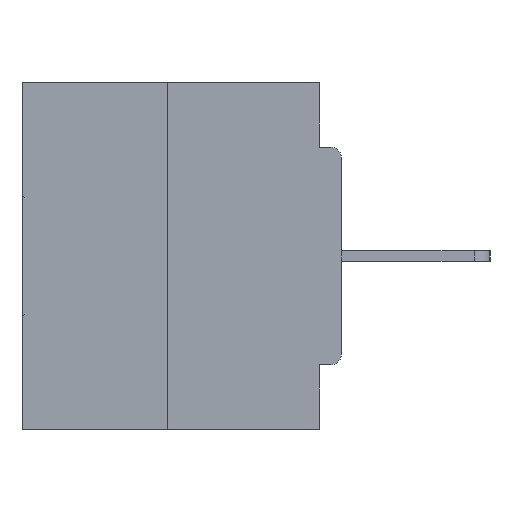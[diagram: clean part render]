
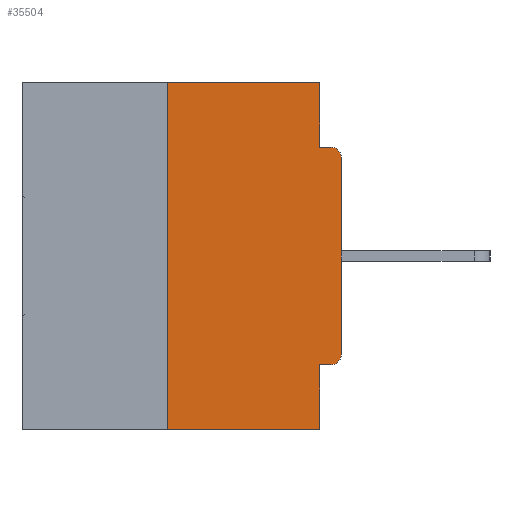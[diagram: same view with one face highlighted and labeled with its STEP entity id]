
A CAD part, left-side view. The second image highlights one B-rep face of the part: STEP entity #35504.
In plain terms, the highlighted planar face has unit normal (-1, 0, 0).
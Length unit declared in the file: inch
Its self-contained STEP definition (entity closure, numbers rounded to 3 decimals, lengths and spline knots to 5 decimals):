
#377 = VECTOR ( 'NONE', #14515, 39.37008 ) ;
#381 = EDGE_CURVE ( 'NONE', #32052, #748, #25562, .T. ) ;
#748 = VERTEX_POINT ( 'NONE', #15202 ) ;
#907 = VERTEX_POINT ( 'NONE', #24732 ) ;
#1870 = ORIENTED_EDGE ( 'NONE', *, *, #14943, .F. ) ;
#2485 = VECTOR ( 'NONE', #12413, 39.37008 ) ;
#2733 = ORIENTED_EDGE ( 'NONE', *, *, #22326, .F. ) ;
#3376 = VECTOR ( 'NONE', #28924, 39.37008 ) ;
#3821 = CARTESIAN_POINT ( 'NONE',  ( 0., 0.015, -0.3915 ) ) ;
#4002 = DIRECTION ( 'NONE',  ( 1., 0., 0. ) ) ;
#4082 = EDGE_CURVE ( 'NONE', #11433, #25136, #16885, .T. ) ;
#5903 = CARTESIAN_POINT ( 'NONE',  ( 0., 0.031, -0.0935 ) ) ;
#6406 = VERTEX_POINT ( 'NONE', #17067 ) ;
#6775 = DIRECTION ( 'NONE',  ( 0., 0., -1. ) ) ;
#7288 = EDGE_CURVE ( 'NONE', #907, #22266, #7903, .T. ) ;
#7825 = ORIENTED_EDGE ( 'NONE', *, *, #21846, .F. ) ;
#7903 = CIRCLE ( 'NONE', #11934, 0.015 ) ;
#8400 = DIRECTION ( 'NONE',  ( 0., -1., 0. ) ) ;
#8404 = ORIENTED_EDGE ( 'NONE', *, *, #32680, .T. ) ;
#8707 = LINE ( 'NONE', #10869, #33222 ) ;
#8786 = CIRCLE ( 'NONE', #23450, 0.015 ) ;
#9446 = EDGE_LOOP ( 'NONE', ( #37067, #15002, #9906, #2733, #30950, #36759, #8404, #12024, #1870, #7825 ) ) ;
#9605 = LINE ( 'NONE', #28944, #32322 ) ;
#9755 = EDGE_CURVE ( 'NONE', #11433, #32052, #9605, .T. ) ;
#9899 = CARTESIAN_POINT ( 'NONE',  ( 0., 0.46, 0. ) ) ;
#9906 = ORIENTED_EDGE ( 'NONE', *, *, #4082, .T. ) ;
#10215 = VERTEX_POINT ( 'NONE', #11180 ) ;
#10403 = VERTEX_POINT ( 'NONE', #5903 ) ;
#10869 = CARTESIAN_POINT ( 'NONE',  ( 0., 0., 0. ) ) ;
#11180 = CARTESIAN_POINT ( 'NONE',  ( 0., 0.015, -0.0935 ) ) ;
#11433 = VERTEX_POINT ( 'NONE', #12003 ) ;
#11456 = CARTESIAN_POINT ( 'NONE',  ( 0., 0.46, 0. ) ) ;
#11932 = VERTEX_POINT ( 'NONE', #14549 ) ;
#11934 = AXIS2_PLACEMENT_3D ( 'NONE', #3821, #24069, #6775 ) ;
#12003 = CARTESIAN_POINT ( 'NONE',  ( 0., 0.25, -0.5 ) ) ;
#12024 = ORIENTED_EDGE ( 'NONE', *, *, #17306, .T. ) ;
#12413 = DIRECTION ( 'NONE',  ( 0., -1., 0. ) ) ;
#12874 = PLANE ( 'NONE',  #25921 ) ;
#13516 = CARTESIAN_POINT ( 'NONE',  ( 0., 0.015, -0.1085 ) ) ;
#14264 = CARTESIAN_POINT ( 'NONE',  ( 0., 0., -0.3915 ) ) ;
#14515 = DIRECTION ( 'NONE',  ( 0., 0., -1. ) ) ;
#14549 = CARTESIAN_POINT ( 'NONE',  ( 0., 0.031, -0.4065 ) ) ;
#14943 = EDGE_CURVE ( 'NONE', #10403, #10215, #35543, .T. ) ;
#15002 = ORIENTED_EDGE ( 'NONE', *, *, #9755, .F. ) ;
#15202 = CARTESIAN_POINT ( 'NONE',  ( 0., 0.031, 0. ) ) ;
#15496 = EDGE_CURVE ( 'NONE', #907, #11932, #19818, .T. ) ;
#15795 = DIRECTION ( 'NONE',  ( 0., 0., -1. ) ) ;
#15974 = VECTOR ( 'NONE', #8400, 39.37008 ) ;
#16427 = DIRECTION ( 'NONE',  ( 0., 0., -1. ) ) ;
#16885 = LINE ( 'NONE', #34002, #15974 ) ;
#17067 = CARTESIAN_POINT ( 'NONE',  ( 0., 0., -0.1085 ) ) ;
#17306 = EDGE_CURVE ( 'NONE', #6406, #10215, #8786, .T. ) ;
#19496 = DIRECTION ( 'NONE',  ( 0., 0., 1. ) ) ;
#19818 = LINE ( 'NONE', #26085, #3376 ) ;
#21846 = EDGE_CURVE ( 'NONE', #748, #10403, #26249, .T. ) ;
#22266 = VERTEX_POINT ( 'NONE', #14264 ) ;
#22326 = EDGE_CURVE ( 'NONE', #11932, #25136, #23577, .T. ) ;
#23450 = AXIS2_PLACEMENT_3D ( 'NONE', #13516, #33257, #16427 ) ;
#23577 = LINE ( 'NONE', #31447, #377 ) ;
#24069 = DIRECTION ( 'NONE',  ( -1., 0., 0. ) ) ;
#24732 = CARTESIAN_POINT ( 'NONE',  ( 0., 0.015, -0.4065 ) ) ;
#25136 = VERTEX_POINT ( 'NONE', #25949 ) ;
#25177 = FACE_OUTER_BOUND ( 'NONE', #9446, .T. ) ;
#25562 = LINE ( 'NONE', #11456, #2485 ) ;
#25921 = AXIS2_PLACEMENT_3D ( 'NONE', #9899, #4002, #15795 ) ;
#25949 = CARTESIAN_POINT ( 'NONE',  ( 0., 0.031, -0.5 ) ) ;
#26085 = CARTESIAN_POINT ( 'NONE',  ( 0., 0., -0.4065 ) ) ;
#26249 = LINE ( 'NONE', #32070, #32790 ) ;
#28238 = VECTOR ( 'NONE', #29329, 39.37008 ) ;
#28835 = DIRECTION ( 'NONE',  ( 0., 0., 1. ) ) ;
#28924 = DIRECTION ( 'NONE',  ( 0., 1., 0. ) ) ;
#28944 = CARTESIAN_POINT ( 'NONE',  ( 0., 0.25, 0. ) ) ;
#29329 = DIRECTION ( 'NONE',  ( 0., -1., 0. ) ) ;
#30352 = CARTESIAN_POINT ( 'NONE',  ( 0., 0.25, 0. ) ) ;
#30950 = ORIENTED_EDGE ( 'NONE', *, *, #15496, .F. ) ;
#31447 = CARTESIAN_POINT ( 'NONE',  ( 0., 0.031, -0.5 ) ) ;
#32052 = VERTEX_POINT ( 'NONE', #30352 ) ;
#32070 = CARTESIAN_POINT ( 'NONE',  ( 0., 0.031, 0. ) ) ;
#32098 = CARTESIAN_POINT ( 'NONE',  ( 0., 0., -0.0935 ) ) ;
#32322 = VECTOR ( 'NONE', #28835, 39.37008 ) ;
#32680 = EDGE_CURVE ( 'NONE', #22266, #6406, #8707, .T. ) ;
#32790 = VECTOR ( 'NONE', #34680, 39.37008 ) ;
#33222 = VECTOR ( 'NONE', #19496, 39.37008 ) ;
#33257 = DIRECTION ( 'NONE',  ( -1., 0., 0. ) ) ;
#34002 = CARTESIAN_POINT ( 'NONE',  ( 0., 0.46, -0.5 ) ) ;
#34680 = DIRECTION ( 'NONE',  ( 0., 0., -1. ) ) ;
#35504 = ADVANCED_FACE ( 'NONE', ( #25177 ), #12874, .F. ) ;
#35543 = LINE ( 'NONE', #32098, #28238 ) ;
#36759 = ORIENTED_EDGE ( 'NONE', *, *, #7288, .T. ) ;
#37067 = ORIENTED_EDGE ( 'NONE', *, *, #381, .F. ) ;
